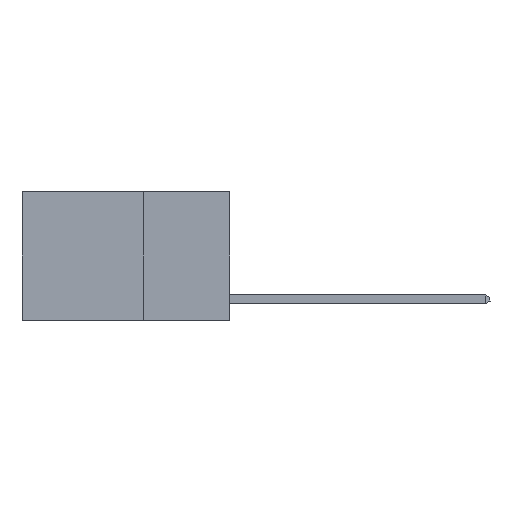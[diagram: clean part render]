
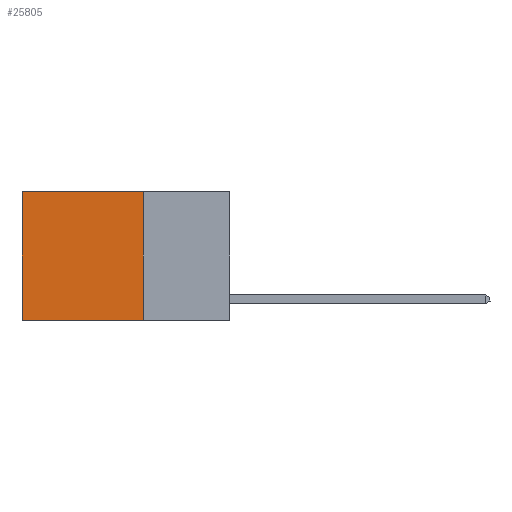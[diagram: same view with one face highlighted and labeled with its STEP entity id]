
A CAD part, left-side view. The second image highlights one B-rep face of the part: STEP entity #25805.
In plain terms, the highlighted planar face has unit normal (-1, 0, 0).
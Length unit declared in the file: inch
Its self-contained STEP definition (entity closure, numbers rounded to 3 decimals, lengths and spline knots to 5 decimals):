
#187 = DIRECTION ( 'NONE',  ( 0., 1., 0. ) ) ;
#320 = CARTESIAN_POINT ( 'NONE',  ( 0.2625, 0.25, 0. ) ) ;
#1508 = CARTESIAN_POINT ( 'NONE',  ( 0.2625, 0.25, 0. ) ) ;
#1528 = DIRECTION ( 'NONE',  ( 0., 0., -1. ) ) ;
#1745 = CARTESIAN_POINT ( 'NONE',  ( 0.2625, 0.25, -0.37 ) ) ;
#2294 = ORIENTED_EDGE ( 'NONE', *, *, #9217, .F. ) ;
#4814 = PLANE ( 'NONE',  #8937 ) ;
#6254 = CARTESIAN_POINT ( 'NONE',  ( 0.2625, 0.6, 0. ) ) ;
#6484 = ORIENTED_EDGE ( 'NONE', *, *, #11372, .F. ) ;
#6585 = CARTESIAN_POINT ( 'NONE',  ( 0.2625, 0.6, -0.37 ) ) ;
#6877 = VERTEX_POINT ( 'NONE', #1508 ) ;
#7209 = DIRECTION ( 'NONE',  ( 1., 0., 0. ) ) ;
#7640 = DIRECTION ( 'NONE',  ( 0., 1., 0. ) ) ;
#8060 = VECTOR ( 'NONE', #1528, 39.37008 ) ;
#8642 = CARTESIAN_POINT ( 'NONE',  ( 0.2625, 0.25, 0. ) ) ;
#8937 = AXIS2_PLACEMENT_3D ( 'NONE', #320, #7209, #15893 ) ;
#9217 = EDGE_CURVE ( 'NONE', #9782, #24550, #13443, .T. ) ;
#9782 = VERTEX_POINT ( 'NONE', #16855 ) ;
#9876 = ORIENTED_EDGE ( 'NONE', *, *, #21344, .T. ) ;
#10159 = CARTESIAN_POINT ( 'NONE',  ( 0.2625, 0.6, 0. ) ) ;
#10851 = DIRECTION ( 'NONE',  ( 0., 0., -1. ) ) ;
#11372 = EDGE_CURVE ( 'NONE', #6877, #9782, #24350, .T. ) ;
#13443 = LINE ( 'NONE', #1745, #17658 ) ;
#15893 = DIRECTION ( 'NONE',  ( 0., 0., -1. ) ) ;
#16855 = CARTESIAN_POINT ( 'NONE',  ( 0.2625, 0.25, -0.37 ) ) ;
#16885 = VECTOR ( 'NONE', #10851, 39.37008 ) ;
#17658 = VECTOR ( 'NONE', #7640, 39.37008 ) ;
#21344 = EDGE_CURVE ( 'NONE', #6877, #28871, #26467, .T. ) ;
#23269 = CARTESIAN_POINT ( 'NONE',  ( 0.2625, 0.25, 0. ) ) ;
#23307 = LINE ( 'NONE', #6254, #16885 ) ;
#23595 = ORIENTED_EDGE ( 'NONE', *, *, #28471, .T. ) ;
#24350 = LINE ( 'NONE', #23269, #8060 ) ;
#24550 = VERTEX_POINT ( 'NONE', #6585 ) ;
#25805 = ADVANCED_FACE ( 'NONE', ( #26321 ), #4814, .F. ) ;
#26321 = FACE_OUTER_BOUND ( 'NONE', #26524, .T. ) ;
#26467 = LINE ( 'NONE', #8642, #28563 ) ;
#26524 = EDGE_LOOP ( 'NONE', ( #23595, #2294, #6484, #9876 ) ) ;
#28471 = EDGE_CURVE ( 'NONE', #28871, #24550, #23307, .T. ) ;
#28563 = VECTOR ( 'NONE', #187, 39.37008 ) ;
#28871 = VERTEX_POINT ( 'NONE', #10159 ) ;
